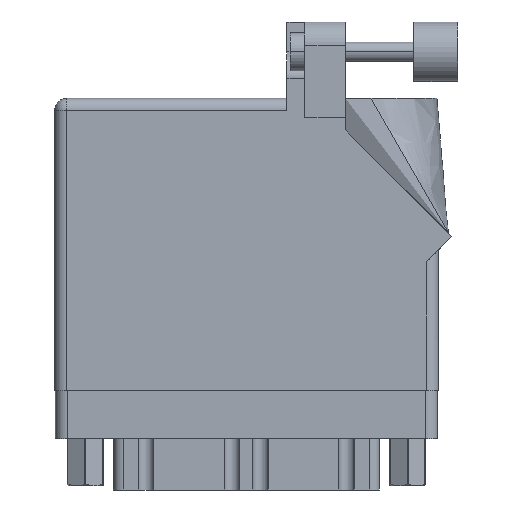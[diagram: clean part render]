
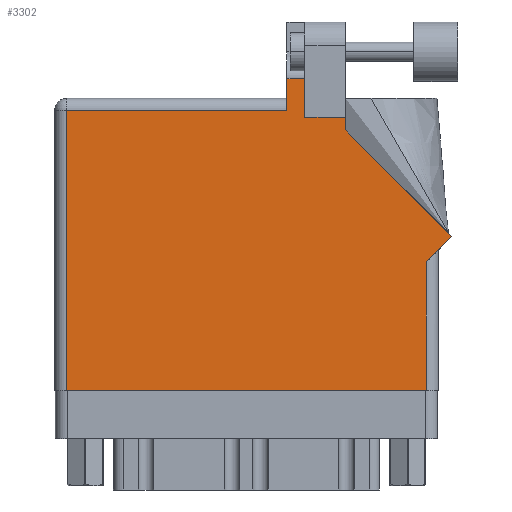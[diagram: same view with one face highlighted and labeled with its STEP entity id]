
A CAD part, front view. The second image highlights one B-rep face of the part: STEP entity #3302.
In plain terms, the highlighted face is planar.
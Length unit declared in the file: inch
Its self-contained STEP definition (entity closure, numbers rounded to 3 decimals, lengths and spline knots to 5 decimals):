
#703 = LINE ( 'NONE', #31370, #23148 ) ;
#835 = CARTESIAN_POINT ( 'NONE',  ( 0.062, 0., 0. ) ) ;
#861 = LINE ( 'NONE', #22869, #45691 ) ;
#1013 = EDGE_CURVE ( 'NONE', #13552, #44136, #30820, .T. ) ;
#1103 = DIRECTION ( 'NONE',  ( 0., 1., 0. ) ) ;
#3179 = CARTESIAN_POINT ( 'NONE',  ( 1.524, 1.36442, 0. ) ) ;
#3302 = ADVANCED_FACE ( 'NONE', ( #27843 ), #16791, .F. ) ;
#3529 = ORIENTED_EDGE ( 'NONE', *, *, #10370, .T. ) ;
#3727 = LINE ( 'NONE', #25949, #47098 ) ;
#4807 = CARTESIAN_POINT ( 'NONE',  ( 0.062, 0., 0. ) ) ;
#4871 = ORIENTED_EDGE ( 'NONE', *, *, #27840, .T. ) ;
#5065 = DIRECTION ( 'NONE',  ( 0.707, 0.707, 0. ) ) ;
#5155 = LINE ( 'NONE', #19902, #28907 ) ;
#6968 = ORIENTED_EDGE ( 'NONE', *, *, #11225, .T. ) ;
#9366 = LINE ( 'NONE', #46102, #21725 ) ;
#9399 = EDGE_CURVE ( 'NONE', #32463, #11304, #703, .T. ) ;
#10370 = EDGE_CURVE ( 'NONE', #29825, #27659, #20646, .T. ) ;
#10872 = VECTOR ( 'NONE', #31000, 39.37008 ) ;
#11225 = EDGE_CURVE ( 'NONE', #33060, #22590, #9366, .T. ) ;
#11304 = VERTEX_POINT ( 'NONE', #20499 ) ;
#11453 = DIRECTION ( 'NONE',  ( -1., 0., 0. ) ) ;
#12627 = VECTOR ( 'NONE', #5065, 39.37008 ) ;
#13552 = VERTEX_POINT ( 'NONE', #17980 ) ;
#14424 = LINE ( 'NONE', #21423, #28359 ) ;
#15848 = DIRECTION ( 'NONE',  ( 0., -1., 0. ) ) ;
#16279 = DIRECTION ( 'NONE',  ( 1., 0., 0. ) ) ;
#16347 = CARTESIAN_POINT ( 'NONE',  ( 1.524, 1.43, 0. ) ) ;
#16762 = CARTESIAN_POINT ( 'NONE',  ( 1.524, 1.36442, 0. ) ) ;
#16791 = PLANE ( 'NONE',  #31160 ) ;
#17030 = DIRECTION ( 'NONE',  ( -1., 0., 0. ) ) ;
#17980 = CARTESIAN_POINT ( 'NONE',  ( 2.08071, 0.80771, 0. ) ) ;
#19484 = CARTESIAN_POINT ( 'NONE',  ( 2.08071, 0.80771, 0. ) ) ;
#19902 = CARTESIAN_POINT ( 'NONE',  ( 0., 0., 0. ) ) ;
#20061 = VERTEX_POINT ( 'NONE', #4807 ) ;
#20377 = DIRECTION ( 'NONE',  ( 0., 0., -1. ) ) ;
#20499 = CARTESIAN_POINT ( 'NONE',  ( 1.311, 1.43, 0. ) ) ;
#20516 = DIRECTION ( 'NONE',  ( -1., 0., 0. ) ) ;
#20591 = ORIENTED_EDGE ( 'NONE', *, *, #1013, .T. ) ;
#20646 = LINE ( 'NONE', #23772, #10872 ) ;
#21178 = DIRECTION ( 'NONE',  ( 0., -1., 0. ) ) ;
#21315 = DIRECTION ( 'NONE',  ( 0., 1., 0. ) ) ;
#21423 = CARTESIAN_POINT ( 'NONE',  ( 1.217, 1.53, 0. ) ) ;
#21541 = CARTESIAN_POINT ( 'NONE',  ( 1.217, 1.6315, 0. ) ) ;
#21725 = VECTOR ( 'NONE', #30639, 39.37008 ) ;
#21887 = CARTESIAN_POINT ( 'NONE',  ( 0.062, 1.468, 0. ) ) ;
#22590 = VERTEX_POINT ( 'NONE', #21887 ) ;
#22637 = ORIENTED_EDGE ( 'NONE', *, *, #33676, .T. ) ;
#22869 = CARTESIAN_POINT ( 'NONE',  ( 1.311, 1.43, 0. ) ) ;
#23148 = VECTOR ( 'NONE', #20516, 39.37008 ) ;
#23772 = CARTESIAN_POINT ( 'NONE',  ( 1.948, 0.737, 0. ) ) ;
#24077 = ORIENTED_EDGE ( 'NONE', *, *, #43127, .T. ) ;
#25261 = VECTOR ( 'NONE', #41690, 39.37008 ) ;
#25949 = CARTESIAN_POINT ( 'NONE',  ( 1.64177, 1.6315, 0. ) ) ;
#26724 = ORIENTED_EDGE ( 'NONE', *, *, #44862, .T. ) ;
#27194 = EDGE_CURVE ( 'NONE', #27659, #13552, #31617, .T. ) ;
#27659 = VERTEX_POINT ( 'NONE', #46211 ) ;
#27741 = CARTESIAN_POINT ( 'NONE',  ( 2.01, 0.737, 0. ) ) ;
#27840 = EDGE_CURVE ( 'NONE', #44136, #32463, #32894, .T. ) ;
#27843 = FACE_OUTER_BOUND ( 'NONE', #39438, .T. ) ;
#28359 = VECTOR ( 'NONE', #21178, 39.37008 ) ;
#28876 = VECTOR ( 'NONE', #21315, 39.37008 ) ;
#28907 = VECTOR ( 'NONE', #16279, 39.37008 ) ;
#29168 = ORIENTED_EDGE ( 'NONE', *, *, #27194, .T. ) ;
#29222 = CARTESIAN_POINT ( 'NONE',  ( 1.217, 1.468, 0. ) ) ;
#29825 = VERTEX_POINT ( 'NONE', #35087 ) ;
#30639 = DIRECTION ( 'NONE',  ( -1., 0., 0. ) ) ;
#30820 = LINE ( 'NONE', #19484, #25261 ) ;
#31000 = DIRECTION ( 'NONE',  ( 0., 1., 0. ) ) ;
#31160 = AXIS2_PLACEMENT_3D ( 'NONE', #46713, #20377, #17030 ) ;
#31370 = CARTESIAN_POINT ( 'NONE',  ( 1.524, 1.43, 0. ) ) ;
#31617 = LINE ( 'NONE', #27741, #12627 ) ;
#32463 = VERTEX_POINT ( 'NONE', #16347 ) ;
#32689 = ORIENTED_EDGE ( 'NONE', *, *, #41901, .T. ) ;
#32894 = LINE ( 'NONE', #3179, #28876 ) ;
#33060 = VERTEX_POINT ( 'NONE', #29222 ) ;
#33327 = VERTEX_POINT ( 'NONE', #45859 ) ;
#33676 = EDGE_CURVE ( 'NONE', #11304, #33327, #861, .T. ) ;
#35087 = CARTESIAN_POINT ( 'NONE',  ( 1.948, 0., 0. ) ) ;
#35414 = VECTOR ( 'NONE', #15848, 39.37008 ) ;
#35823 = ORIENTED_EDGE ( 'NONE', *, *, #9399, .T. ) ;
#36167 = EDGE_CURVE ( 'NONE', #20061, #29825, #5155, .T. ) ;
#38986 = ORIENTED_EDGE ( 'NONE', *, *, #36167, .T. ) ;
#39438 = EDGE_LOOP ( 'NONE', ( #22637, #26724, #32689, #6968, #24077, #38986, #3529, #29168, #20591, #4871, #35823 ) ) ;
#41690 = DIRECTION ( 'NONE',  ( -0.707, 0.707, 0. ) ) ;
#41901 = EDGE_CURVE ( 'NONE', #44315, #33060, #14424, .T. ) ;
#43127 = EDGE_CURVE ( 'NONE', #22590, #20061, #44589, .T. ) ;
#44136 = VERTEX_POINT ( 'NONE', #16762 ) ;
#44315 = VERTEX_POINT ( 'NONE', #21541 ) ;
#44589 = LINE ( 'NONE', #835, #35414 ) ;
#44862 = EDGE_CURVE ( 'NONE', #33327, #44315, #3727, .T. ) ;
#45691 = VECTOR ( 'NONE', #1103, 39.37008 ) ;
#45859 = CARTESIAN_POINT ( 'NONE',  ( 1.311, 1.6315, 0. ) ) ;
#46102 = CARTESIAN_POINT ( 'NONE',  ( 0., 1.468, 0. ) ) ;
#46211 = CARTESIAN_POINT ( 'NONE',  ( 1.948, 0.675, 0. ) ) ;
#46713 = CARTESIAN_POINT ( 'NONE',  ( 0., 1.53, 0. ) ) ;
#47098 = VECTOR ( 'NONE', #11453, 39.37008 ) ;
